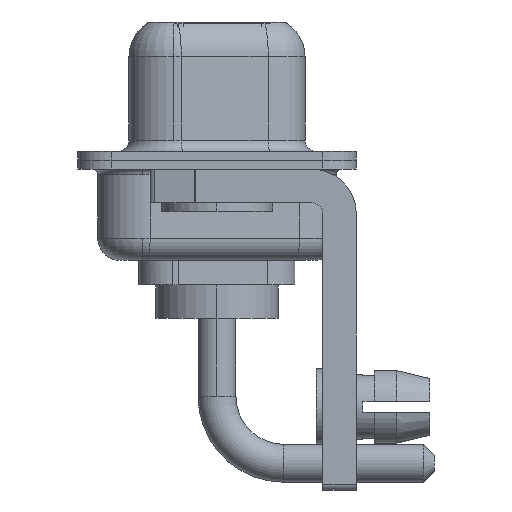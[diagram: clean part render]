
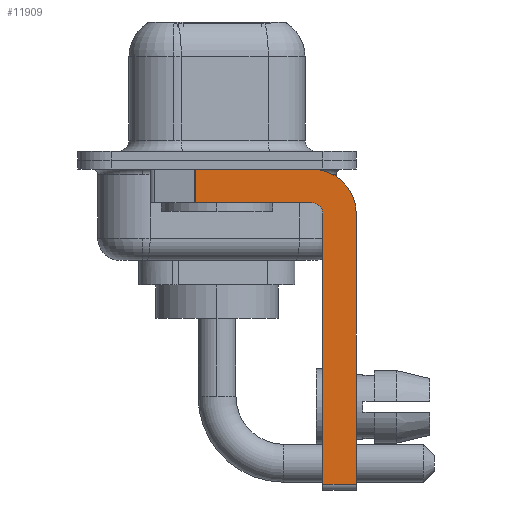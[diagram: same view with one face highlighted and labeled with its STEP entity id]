
A CAD part, left-side view. The second image highlights one B-rep face of the part: STEP entity #11909.
In plain terms, the highlighted planar face has unit normal (-1, 0, 0).
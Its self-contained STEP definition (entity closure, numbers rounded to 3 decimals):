
#1817 = DIRECTION ( 'NONE',  ( 1., 0., 0. ) ) ;
#1851 = ORIENTED_EDGE ( 'NONE', *, *, #13816, .F. ) ;
#1870 = VERTEX_POINT ( 'NONE', #2296 ) ;
#2296 = CARTESIAN_POINT ( 'NONE',  ( -2.9, -4.25, -0.4 ) ) ;
#2544 = VECTOR ( 'NONE', #12852, 1000. ) ;
#2643 = CARTESIAN_POINT ( 'NONE',  ( -2.9, -4.75, -2.4 ) ) ;
#2724 = CARTESIAN_POINT ( 'NONE',  ( -2.9, -6.25, -2.4 ) ) ;
#2830 = AXIS2_PLACEMENT_3D ( 'NONE', #8882, #13549, #9187 ) ;
#3004 = DIRECTION ( 'NONE',  ( 0., -1., 0. ) ) ;
#3768 = ORIENTED_EDGE ( 'NONE', *, *, #6935, .F. ) ;
#4053 = VECTOR ( 'NONE', #6089, 1000. ) ;
#4205 = FACE_OUTER_BOUND ( 'NONE', #5062, .T. ) ;
#4490 = EDGE_CURVE ( 'NONE', #10694, #6064, #12084, .T. ) ;
#4858 = EDGE_CURVE ( 'NONE', #9031, #7113, #5932, .T. ) ;
#5062 = EDGE_LOOP ( 'NONE', ( #1851, #6228, #5122, #3768, #7554, #13814, #7148, #11582 ) ) ;
#5122 = ORIENTED_EDGE ( 'NONE', *, *, #10220, .F. ) ;
#5175 = CARTESIAN_POINT ( 'NONE',  ( -2.9, -4.25, -1.9 ) ) ;
#5329 = DIRECTION ( 'NONE',  ( 0., 0., -1. ) ) ;
#5565 = LINE ( 'NONE', #7633, #8455 ) ;
#5932 = LINE ( 'NONE', #12749, #7871 ) ;
#6017 = CIRCLE ( 'NONE', #11634, 2. ) ;
#6064 = VERTEX_POINT ( 'NONE', #8724 ) ;
#6089 = DIRECTION ( 'NONE',  ( 0., 0., -1. ) ) ;
#6228 = ORIENTED_EDGE ( 'NONE', *, *, #4858, .T. ) ;
#6397 = VERTEX_POINT ( 'NONE', #5175 ) ;
#6401 = EDGE_CURVE ( 'NONE', #10694, #10899, #11851, .T. ) ;
#6456 = AXIS2_PLACEMENT_3D ( 'NONE', #13555, #7740, #7665 ) ;
#6935 = EDGE_CURVE ( 'NONE', #10899, #6397, #7671, .T. ) ;
#7113 = VERTEX_POINT ( 'NONE', #9416 ) ;
#7148 = ORIENTED_EDGE ( 'NONE', *, *, #13204, .F. ) ;
#7201 = CARTESIAN_POINT ( 'NONE',  ( -2.9, 0.978, -0.4 ) ) ;
#7264 = CARTESIAN_POINT ( 'NONE',  ( -2.9, -6.25, -2.4 ) ) ;
#7554 = ORIENTED_EDGE ( 'NONE', *, *, #6401, .F. ) ;
#7587 = CARTESIAN_POINT ( 'NONE',  ( -2.9, 3., -0.4 ) ) ;
#7633 = CARTESIAN_POINT ( 'NONE',  ( -2.9, -4.25, -1.9 ) ) ;
#7665 = DIRECTION ( 'NONE',  ( 0., 0., 1. ) ) ;
#7671 = CIRCLE ( 'NONE', #6456, 0.5 ) ;
#7684 = VERTEX_POINT ( 'NONE', #7264 ) ;
#7740 = DIRECTION ( 'NONE',  ( -1., 0., 0. ) ) ;
#7871 = VECTOR ( 'NONE', #10604, 1000. ) ;
#8455 = VECTOR ( 'NONE', #8934, 1000. ) ;
#8481 = DIRECTION ( 'NONE',  ( 0., -1., 0. ) ) ;
#8615 = LINE ( 'NONE', #2724, #4053 ) ;
#8724 = CARTESIAN_POINT ( 'NONE',  ( -2.9, -6.25, -14.55 ) ) ;
#8882 = CARTESIAN_POINT ( 'NONE',  ( -2.9, -4.25, -2.4 ) ) ;
#8934 = DIRECTION ( 'NONE',  ( 0., 1., 0. ) ) ;
#8961 = PLANE ( 'NONE',  #2830 ) ;
#9031 = VERTEX_POINT ( 'NONE', #7201 ) ;
#9187 = DIRECTION ( 'NONE',  ( 0., 0., -1. ) ) ;
#9416 = CARTESIAN_POINT ( 'NONE',  ( -2.9, 0.978, -1.9 ) ) ;
#9839 = CARTESIAN_POINT ( 'NONE',  ( -2.9, -4.75, -14.55 ) ) ;
#10220 = EDGE_CURVE ( 'NONE', #6397, #7113, #5565, .T. ) ;
#10604 = DIRECTION ( 'NONE',  ( 0., 0., -1. ) ) ;
#10651 = EDGE_CURVE ( 'NONE', #1870, #7684, #6017, .T. ) ;
#10694 = VERTEX_POINT ( 'NONE', #9839 ) ;
#10899 = VERTEX_POINT ( 'NONE', #2643 ) ;
#10925 = CARTESIAN_POINT ( 'NONE',  ( -2.9, -4.25, -14.55 ) ) ;
#11039 = LINE ( 'NONE', #7587, #13809 ) ;
#11059 = CARTESIAN_POINT ( 'NONE',  ( -2.9, -4.75, -14.8 ) ) ;
#11280 = VECTOR ( 'NONE', #8481, 1000. ) ;
#11582 = ORIENTED_EDGE ( 'NONE', *, *, #10651, .F. ) ;
#11634 = AXIS2_PLACEMENT_3D ( 'NONE', #12302, #1817, #5329 ) ;
#11851 = LINE ( 'NONE', #11059, #2544 ) ;
#11909 = ADVANCED_FACE ( 'NONE', ( #4205 ), #8961, .F. ) ;
#12084 = LINE ( 'NONE', #10925, #11280 ) ;
#12302 = CARTESIAN_POINT ( 'NONE',  ( -2.9, -4.25, -2.4 ) ) ;
#12749 = CARTESIAN_POINT ( 'NONE',  ( -2.9, 0.978, -1.9 ) ) ;
#12852 = DIRECTION ( 'NONE',  ( 0., 0., 1. ) ) ;
#13204 = EDGE_CURVE ( 'NONE', #7684, #6064, #8615, .T. ) ;
#13549 = DIRECTION ( 'NONE',  ( 1., 0., 0. ) ) ;
#13555 = CARTESIAN_POINT ( 'NONE',  ( -2.9, -4.25, -2.4 ) ) ;
#13809 = VECTOR ( 'NONE', #3004, 1000. ) ;
#13814 = ORIENTED_EDGE ( 'NONE', *, *, #4490, .T. ) ;
#13816 = EDGE_CURVE ( 'NONE', #9031, #1870, #11039, .T. ) ;
